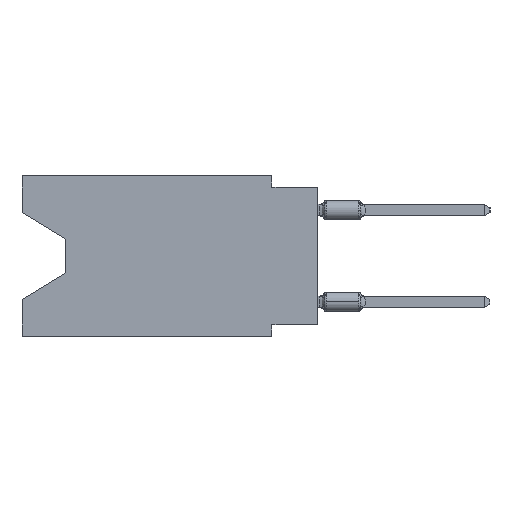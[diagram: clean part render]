
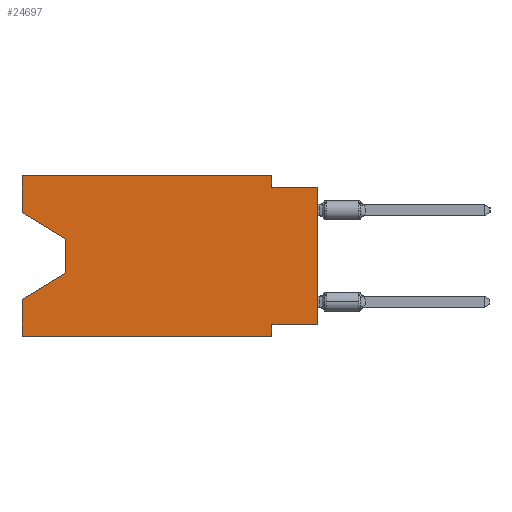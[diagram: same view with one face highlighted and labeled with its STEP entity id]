
A CAD part, left-side view. The second image highlights one B-rep face of the part: STEP entity #24697.
In plain terms, the highlighted planar face has unit normal (-1, 0, 0).
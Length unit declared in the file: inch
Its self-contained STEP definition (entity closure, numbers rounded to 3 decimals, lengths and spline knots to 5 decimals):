
#67 = EDGE_CURVE ( 'NONE', #39158, #16511, #9344, .T. ) ;
#823 = ORIENTED_EDGE ( 'NONE', *, *, #38340, .F. ) ;
#972 = CARTESIAN_POINT ( 'NONE',  ( 0., 0., -0.025 ) ) ;
#1005 = CARTESIAN_POINT ( 'NONE',  ( 0., 0.645, 0. ) ) ;
#3366 = EDGE_CURVE ( 'NONE', #43081, #25166, #37733, .T. ) ;
#4454 = ORIENTED_EDGE ( 'NONE', *, *, #5118, .F. ) ;
#4895 = CARTESIAN_POINT ( 'NONE',  ( 0., 0.645, 0. ) ) ;
#4896 = DIRECTION ( 'NONE',  ( 0., 0.855, -0.519 ) ) ;
#5118 = EDGE_CURVE ( 'NONE', #7730, #39158, #32903, .T. ) ;
#5412 = DIRECTION ( 'NONE',  ( 0., -1., 0. ) ) ;
#6046 = DIRECTION ( 'NONE',  ( 0., 1., 0. ) ) ;
#7165 = VERTEX_POINT ( 'NONE', #31074 ) ;
#7403 = LINE ( 'NONE', #15331, #21362 ) ;
#7730 = VERTEX_POINT ( 'NONE', #47825 ) ;
#8489 = LINE ( 'NONE', #12308, #11384 ) ;
#9344 = LINE ( 'NONE', #40054, #28901 ) ;
#10710 = CARTESIAN_POINT ( 'NONE',  ( 0., 0.645, -0.26975 ) ) ;
#10788 = ORIENTED_EDGE ( 'NONE', *, *, #48641, .T. ) ;
#10873 = ORIENTED_EDGE ( 'NONE', *, *, #24874, .T. ) ;
#11009 = VECTOR ( 'NONE', #6046, 39.37008 ) ;
#11384 = VECTOR ( 'NONE', #5412, 39.37008 ) ;
#11500 = VERTEX_POINT ( 'NONE', #38557 ) ;
#11554 = VECTOR ( 'NONE', #14702, 39.37008 ) ;
#11746 = ORIENTED_EDGE ( 'NONE', *, *, #39386, .T. ) ;
#11924 = CARTESIAN_POINT ( 'NONE',  ( 0., 0.55, -0.212 ) ) ;
#12065 = EDGE_CURVE ( 'NONE', #11500, #33300, #21983, .T. ) ;
#12068 = CARTESIAN_POINT ( 'NONE',  ( 0., 0.1, -0.025 ) ) ;
#12308 = CARTESIAN_POINT ( 'NONE',  ( 0., 0.645, 0. ) ) ;
#13126 = EDGE_CURVE ( 'NONE', #7165, #29117, #8489, .T. ) ;
#14685 = ORIENTED_EDGE ( 'NONE', *, *, #28110, .T. ) ;
#14702 = DIRECTION ( 'NONE',  ( 0., -1., 0. ) ) ;
#14924 = EDGE_CURVE ( 'NONE', #29117, #43081, #37830, .T. ) ;
#15331 = CARTESIAN_POINT ( 'NONE',  ( 0., 0.645, -0.08025 ) ) ;
#16079 = ORIENTED_EDGE ( 'NONE', *, *, #67, .F. ) ;
#16511 = VERTEX_POINT ( 'NONE', #22227 ) ;
#17190 = CARTESIAN_POINT ( 'NONE',  ( 0., 0., 0. ) ) ;
#17751 = CARTESIAN_POINT ( 'NONE',  ( 0., 0., -0.025 ) ) ;
#17829 = VECTOR ( 'NONE', #41938, 39.37008 ) ;
#17876 = VECTOR ( 'NONE', #37404, 39.37008 ) ;
#20238 = PLANE ( 'NONE',  #43303 ) ;
#20492 = DIRECTION ( 'NONE',  ( 1., 0., 0. ) ) ;
#21021 = FACE_OUTER_BOUND ( 'NONE', #30190, .T. ) ;
#21054 = CARTESIAN_POINT ( 'NONE',  ( 0., 0.1, 0. ) ) ;
#21362 = VECTOR ( 'NONE', #22988, 39.37008 ) ;
#21983 = LINE ( 'NONE', #45775, #17829 ) ;
#22227 = CARTESIAN_POINT ( 'NONE',  ( 0., 0.1, -0.35 ) ) ;
#22988 = DIRECTION ( 'NONE',  ( 0., -0.855, -0.519 ) ) ;
#23555 = LINE ( 'NONE', #1005, #44283 ) ;
#23951 = VERTEX_POINT ( 'NONE', #38960 ) ;
#24358 = LINE ( 'NONE', #48401, #27693 ) ;
#24370 = DIRECTION ( 'NONE',  ( 0., 0., 1. ) ) ;
#24461 = CARTESIAN_POINT ( 'NONE',  ( 0., 0.55, -0.138 ) ) ;
#24697 = ADVANCED_FACE ( 'NONE', ( #21021 ), #20238, .F. ) ;
#24874 = EDGE_CURVE ( 'NONE', #11500, #16511, #33285, .T. ) ;
#24886 = LINE ( 'NONE', #17190, #27027 ) ;
#25166 = VERTEX_POINT ( 'NONE', #972 ) ;
#25200 = DIRECTION ( 'NONE',  ( 0., 0., -1. ) ) ;
#25558 = CARTESIAN_POINT ( 'NONE',  ( 0., 0.1, 0. ) ) ;
#27027 = VECTOR ( 'NONE', #24370, 39.37008 ) ;
#27237 = EDGE_CURVE ( 'NONE', #7730, #25166, #24886, .T. ) ;
#27693 = VECTOR ( 'NONE', #4896, 39.37008 ) ;
#28033 = DIRECTION ( 'NONE',  ( 0., 0., -1. ) ) ;
#28110 = EDGE_CURVE ( 'NONE', #29228, #23951, #7403, .T. ) ;
#28182 = DIRECTION ( 'NONE',  ( 0., 0., -1. ) ) ;
#28901 = VECTOR ( 'NONE', #25200, 39.37008 ) ;
#29117 = VERTEX_POINT ( 'NONE', #21054 ) ;
#29228 = VERTEX_POINT ( 'NONE', #41272 ) ;
#29703 = CARTESIAN_POINT ( 'NONE',  ( 0., 0.645, -0.35 ) ) ;
#29781 = ORIENTED_EDGE ( 'NONE', *, *, #3366, .F. ) ;
#29813 = CARTESIAN_POINT ( 'NONE',  ( 0., 0., -0.325 ) ) ;
#30190 = EDGE_LOOP ( 'NONE', ( #14685, #11746, #10788, #33023, #10873, #16079, #4454, #41204, #29781, #35191, #44603, #823 ) ) ;
#30624 = CARTESIAN_POINT ( 'NONE',  ( 0., 0.1, -0.325 ) ) ;
#31006 = VECTOR ( 'NONE', #40922, 39.37008 ) ;
#31074 = CARTESIAN_POINT ( 'NONE',  ( 0., 0.645, 0. ) ) ;
#31748 = DIRECTION ( 'NONE',  ( 0., 0., 1. ) ) ;
#32903 = LINE ( 'NONE', #29813, #11009 ) ;
#33023 = ORIENTED_EDGE ( 'NONE', *, *, #12065, .F. ) ;
#33285 = LINE ( 'NONE', #29703, #17876 ) ;
#33300 = VERTEX_POINT ( 'NONE', #10710 ) ;
#34498 = VECTOR ( 'NONE', #28033, 39.37008 ) ;
#35191 = ORIENTED_EDGE ( 'NONE', *, *, #14924, .F. ) ;
#37404 = DIRECTION ( 'NONE',  ( 0., -1., 0. ) ) ;
#37733 = LINE ( 'NONE', #17751, #11554 ) ;
#37830 = LINE ( 'NONE', #25558, #31006 ) ;
#38340 = EDGE_CURVE ( 'NONE', #29228, #7165, #23555, .T. ) ;
#38557 = CARTESIAN_POINT ( 'NONE',  ( 0., 0.645, -0.35 ) ) ;
#38960 = CARTESIAN_POINT ( 'NONE',  ( 0., 0.55, -0.138 ) ) ;
#39158 = VERTEX_POINT ( 'NONE', #30624 ) ;
#39386 = EDGE_CURVE ( 'NONE', #23951, #41011, #48755, .T. ) ;
#40054 = CARTESIAN_POINT ( 'NONE',  ( 0., 0.1, -0.35 ) ) ;
#40922 = DIRECTION ( 'NONE',  ( 0., 0., -1. ) ) ;
#41011 = VERTEX_POINT ( 'NONE', #11924 ) ;
#41204 = ORIENTED_EDGE ( 'NONE', *, *, #27237, .T. ) ;
#41272 = CARTESIAN_POINT ( 'NONE',  ( 0., 0.645, -0.08025 ) ) ;
#41938 = DIRECTION ( 'NONE',  ( 0., 0., 1. ) ) ;
#43081 = VERTEX_POINT ( 'NONE', #12068 ) ;
#43303 = AXIS2_PLACEMENT_3D ( 'NONE', #4895, #20492, #28182 ) ;
#44283 = VECTOR ( 'NONE', #31748, 39.37008 ) ;
#44603 = ORIENTED_EDGE ( 'NONE', *, *, #13126, .F. ) ;
#45775 = CARTESIAN_POINT ( 'NONE',  ( 0., 0.645, 0. ) ) ;
#47825 = CARTESIAN_POINT ( 'NONE',  ( 0., 0., -0.325 ) ) ;
#48401 = CARTESIAN_POINT ( 'NONE',  ( 0., 0.55, -0.212 ) ) ;
#48641 = EDGE_CURVE ( 'NONE', #41011, #33300, #24358, .T. ) ;
#48755 = LINE ( 'NONE', #24461, #34498 ) ;
